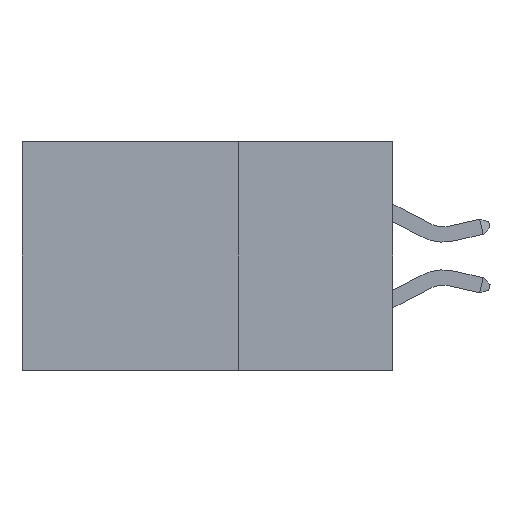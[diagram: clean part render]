
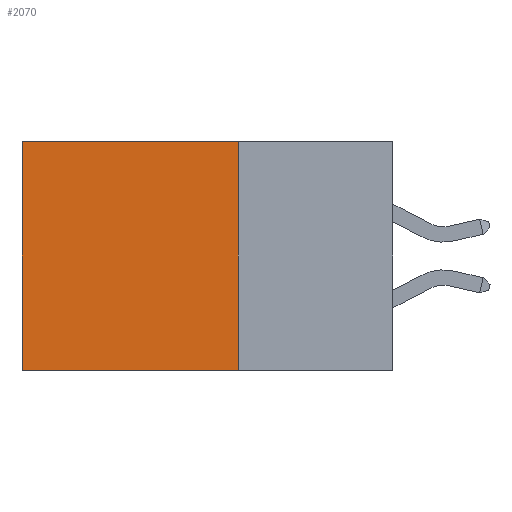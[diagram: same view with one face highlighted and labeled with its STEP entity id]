
A CAD part, left-side view. The second image highlights one B-rep face of the part: STEP entity #2070.
In plain terms, the highlighted planar face has unit normal (-1, 0, 0).
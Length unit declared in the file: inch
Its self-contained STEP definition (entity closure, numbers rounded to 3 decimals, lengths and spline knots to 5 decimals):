
#2070 = ADVANCED_FACE ( 'NONE', ( #14728 ), #14548, .F. ) ;
#2642 = EDGE_LOOP ( 'NONE', ( #15233, #4349, #11831, #5618 ) ) ;
#2902 = DIRECTION ( 'NONE',  ( 0., 1., 0. ) ) ;
#4145 = DIRECTION ( 'NONE',  ( 0., 0., -1. ) ) ;
#4349 = ORIENTED_EDGE ( 'NONE', *, *, #8713, .F. ) ;
#5618 = ORIENTED_EDGE ( 'NONE', *, *, #13336, .T. ) ;
#5693 = LINE ( 'NONE', #9308, #6939 ) ;
#6124 = DIRECTION ( 'NONE',  ( 0., 0., -1. ) ) ;
#6423 = VECTOR ( 'NONE', #8721, 39.37008 ) ;
#6908 = EDGE_CURVE ( 'NONE', #9383, #10372, #12097, .T. ) ;
#6939 = VECTOR ( 'NONE', #4145, 39.37008 ) ;
#7091 = CARTESIAN_POINT ( 'NONE',  ( 0.2875, 0.6, 0. ) ) ;
#7769 = VECTOR ( 'NONE', #2902, 39.37008 ) ;
#8059 = DIRECTION ( 'NONE',  ( 1., 0., 0. ) ) ;
#8102 = VERTEX_POINT ( 'NONE', #8570 ) ;
#8570 = CARTESIAN_POINT ( 'NONE',  ( 0.2875, 0.25, -0.37 ) ) ;
#8629 = AXIS2_PLACEMENT_3D ( 'NONE', #15867, #8059, #10689 ) ;
#8713 = EDGE_CURVE ( 'NONE', #8102, #10372, #15309, .T. ) ;
#8721 = DIRECTION ( 'NONE',  ( 0., 1., 0. ) ) ;
#8897 = CARTESIAN_POINT ( 'NONE',  ( 0.2875, 0.25, 0. ) ) ;
#8908 = LINE ( 'NONE', #8897, #6423 ) ;
#9308 = CARTESIAN_POINT ( 'NONE',  ( 0.2875, 0.25, 0. ) ) ;
#9383 = VERTEX_POINT ( 'NONE', #7091 ) ;
#9988 = CARTESIAN_POINT ( 'NONE',  ( 0.2875, 0.6, 0. ) ) ;
#10372 = VERTEX_POINT ( 'NONE', #12471 ) ;
#10689 = DIRECTION ( 'NONE',  ( 0., 0., -1. ) ) ;
#11005 = CARTESIAN_POINT ( 'NONE',  ( 0.2875, 0.25, -0.37 ) ) ;
#11156 = VERTEX_POINT ( 'NONE', #12782 ) ;
#11831 = ORIENTED_EDGE ( 'NONE', *, *, #16783, .F. ) ;
#12097 = LINE ( 'NONE', #9988, #15765 ) ;
#12471 = CARTESIAN_POINT ( 'NONE',  ( 0.2875, 0.6, -0.37 ) ) ;
#12782 = CARTESIAN_POINT ( 'NONE',  ( 0.2875, 0.25, 0. ) ) ;
#13336 = EDGE_CURVE ( 'NONE', #11156, #9383, #8908, .T. ) ;
#14548 = PLANE ( 'NONE',  #8629 ) ;
#14728 = FACE_OUTER_BOUND ( 'NONE', #2642, .T. ) ;
#15233 = ORIENTED_EDGE ( 'NONE', *, *, #6908, .T. ) ;
#15309 = LINE ( 'NONE', #11005, #7769 ) ;
#15765 = VECTOR ( 'NONE', #6124, 39.37008 ) ;
#15867 = CARTESIAN_POINT ( 'NONE',  ( 0.2875, 0.25, 0. ) ) ;
#16783 = EDGE_CURVE ( 'NONE', #11156, #8102, #5693, .T. ) ;
